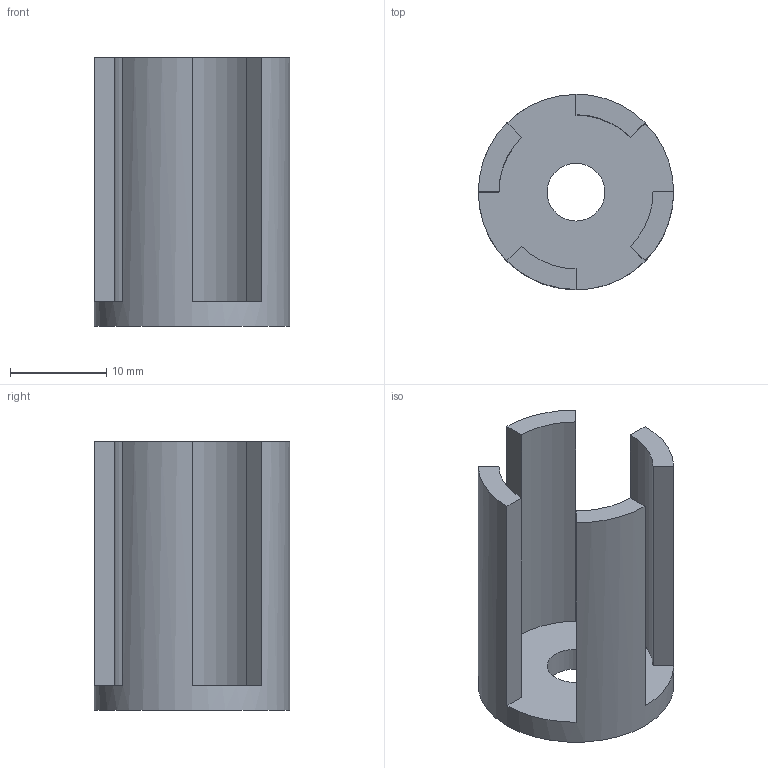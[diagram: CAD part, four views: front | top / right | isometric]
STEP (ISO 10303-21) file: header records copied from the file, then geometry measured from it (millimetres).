
FILE_DESCRIPTION(/* description */ (''),/* implementation_level */ '2;1');
FILE_NAME(/* name */ 'End Pilot for 6mm Rod.stp',/* time_stamp */ '2019-12-05T11:03:28-06:00',/* author */ ('johne'),/* organization */ (''),/* preprocessor_version */ 'ST-DEVELOPER v18',/* originating_system */ 'Autodesk Inventor 2020',/* authorisation */ '');
FILE_SCHEMA (('AUTOMOTIVE_DESIGN { 1 0 10303 214 3 1 1 }'));
Length unit declared in the file: inch
Products named in the file (1): End Pilot for 6mm Rod
Bounding box: 20.32 x 20.32 x 27.94 mm (x, y, z)
Volume: 2310.4 mm3; surface area: 2688.8 mm2
Topology: 1 solids, 1 shells, 20 faces, 53 edges, 35 vertices
Faces by surface type: plane 14, cylinder 6
Full cylindrical faces by diameter (mm): 6.005 x1, 20.32 x1
Entity records: 675 total; most frequent: DIRECTION 114, CARTESIAN_POINT 109, ORIENTED_EDGE 106, EDGE_CURVE 53, AXIS2_PLACEMENT_3D 40, VERTEX_POINT 35, LINE 34, VECTOR 34
